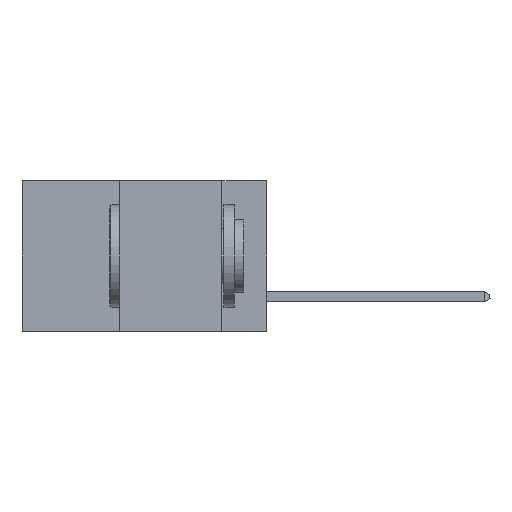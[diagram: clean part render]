
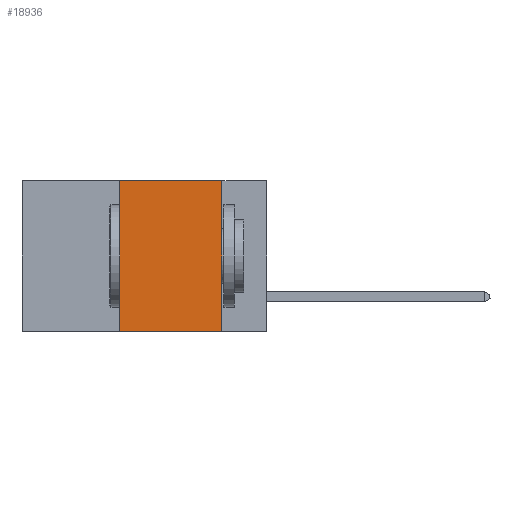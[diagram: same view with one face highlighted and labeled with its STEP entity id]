
A CAD part, left-side view. The second image highlights one B-rep face of the part: STEP entity #18936.
In plain terms, the highlighted planar face has unit normal (-1, 0, 0).
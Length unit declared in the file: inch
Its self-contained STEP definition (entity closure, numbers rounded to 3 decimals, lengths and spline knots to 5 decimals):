
#700 = LINE ( 'NONE', #16180, #17631 ) ;
#1794 = VECTOR ( 'NONE', #20254, 39.37008 ) ;
#3718 = CARTESIAN_POINT ( 'NONE',  ( 0., 0.11, 0. ) ) ;
#3939 = DIRECTION ( 'NONE',  ( 0., -1., 0. ) ) ;
#4290 = CARTESIAN_POINT ( 'NONE',  ( 0., 0.36, 0. ) ) ;
#5300 = VERTEX_POINT ( 'NONE', #4290 ) ;
#6232 = EDGE_CURVE ( 'NONE', #16028, #5300, #13094, .T. ) ;
#6652 = LINE ( 'NONE', #3718, #1794 ) ;
#6943 = CARTESIAN_POINT ( 'NONE',  ( 0., 0.11, 0. ) ) ;
#7910 = VECTOR ( 'NONE', #9151, 39.37008 ) ;
#8005 = PLANE ( 'NONE',  #15505 ) ;
#9151 = DIRECTION ( 'NONE',  ( 0., 0., 1. ) ) ;
#9374 = ORIENTED_EDGE ( 'NONE', *, *, #16204, .T. ) ;
#9507 = VERTEX_POINT ( 'NONE', #6943 ) ;
#9789 = CARTESIAN_POINT ( 'NONE',  ( 0., 0.6, 0. ) ) ;
#10016 = CARTESIAN_POINT ( 'NONE',  ( 0., 0.36, 0. ) ) ;
#10175 = CARTESIAN_POINT ( 'NONE',  ( 0., 0.36, -0.37 ) ) ;
#10184 = ORIENTED_EDGE ( 'NONE', *, *, #11931, .F. ) ;
#11931 = EDGE_CURVE ( 'NONE', #5300, #9507, #15446, .T. ) ;
#13094 = LINE ( 'NONE', #10016, #7910 ) ;
#14630 = EDGE_LOOP ( 'NONE', ( #20916, #10184, #19989, #9374 ) ) ;
#15446 = LINE ( 'NONE', #18733, #16298 ) ;
#15505 = AXIS2_PLACEMENT_3D ( 'NONE', #9789, #18957, #15558 ) ;
#15558 = DIRECTION ( 'NONE',  ( 0., 0., -1. ) ) ;
#16028 = VERTEX_POINT ( 'NONE', #10175 ) ;
#16180 = CARTESIAN_POINT ( 'NONE',  ( 0., 0.6, -0.37 ) ) ;
#16204 = EDGE_CURVE ( 'NONE', #16028, #18618, #700, .T. ) ;
#16298 = VECTOR ( 'NONE', #3939, 39.37008 ) ;
#17631 = VECTOR ( 'NONE', #19737, 39.37008 ) ;
#18618 = VERTEX_POINT ( 'NONE', #21427 ) ;
#18733 = CARTESIAN_POINT ( 'NONE',  ( 0., 0.6, 0. ) ) ;
#18936 = ADVANCED_FACE ( 'NONE', ( #23588 ), #8005, .F. ) ;
#18957 = DIRECTION ( 'NONE',  ( 1., 0., 0. ) ) ;
#19737 = DIRECTION ( 'NONE',  ( 0., -1., 0. ) ) ;
#19989 = ORIENTED_EDGE ( 'NONE', *, *, #6232, .F. ) ;
#20032 = EDGE_CURVE ( 'NONE', #9507, #18618, #6652, .T. ) ;
#20254 = DIRECTION ( 'NONE',  ( 0., 0., -1. ) ) ;
#20916 = ORIENTED_EDGE ( 'NONE', *, *, #20032, .F. ) ;
#21427 = CARTESIAN_POINT ( 'NONE',  ( 0., 0.11, -0.37 ) ) ;
#23588 = FACE_OUTER_BOUND ( 'NONE', #14630, .T. ) ;
